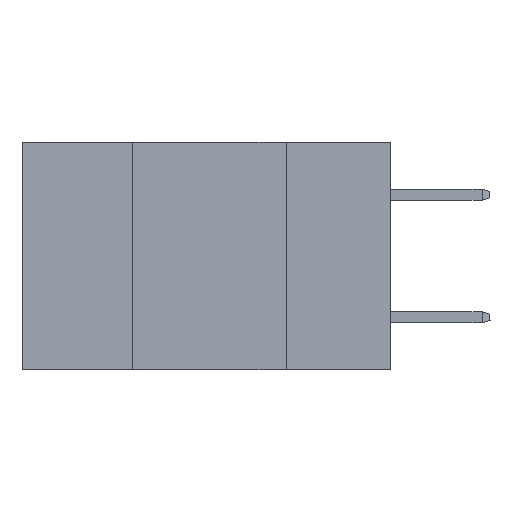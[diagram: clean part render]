
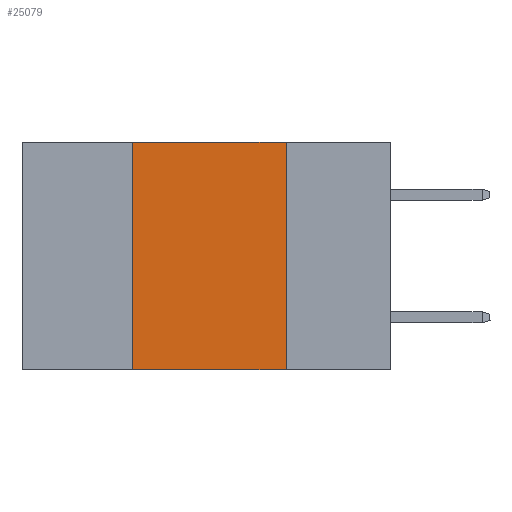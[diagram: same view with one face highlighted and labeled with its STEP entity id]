
A CAD part, left-side view. The second image highlights one B-rep face of the part: STEP entity #25079.
In plain terms, the highlighted planar face has unit normal (-1, 0, 0).
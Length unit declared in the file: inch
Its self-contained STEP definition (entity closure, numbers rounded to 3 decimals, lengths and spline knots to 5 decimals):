
#1351 = ORIENTED_EDGE ( 'NONE', *, *, #25107, .T. ) ;
#2371 = VECTOR ( 'NONE', #12597, 39.37008 ) ;
#2726 = PLANE ( 'NONE',  #24938 ) ;
#3390 = DIRECTION ( 'NONE',  ( 0., 0., -1. ) ) ;
#3942 = ORIENTED_EDGE ( 'NONE', *, *, #21817, .F. ) ;
#7204 = CARTESIAN_POINT ( 'NONE',  ( 0., 0.6, 0. ) ) ;
#9148 = DIRECTION ( 'NONE',  ( 0., -1., 0. ) ) ;
#9294 = LINE ( 'NONE', #16383, #20181 ) ;
#9802 = EDGE_LOOP ( 'NONE', ( #15113, #3942, #19496, #1351 ) ) ;
#12597 = DIRECTION ( 'NONE',  ( 0., 0., 1. ) ) ;
#13269 = CARTESIAN_POINT ( 'NONE',  ( 0., 0.6, 0. ) ) ;
#13575 = LINE ( 'NONE', #17907, #27527 ) ;
#14464 = VERTEX_POINT ( 'NONE', #16578 ) ;
#14488 = EDGE_CURVE ( 'NONE', #17779, #22284, #9294, .T. ) ;
#15113 = ORIENTED_EDGE ( 'NONE', *, *, #14488, .F. ) ;
#15718 = DIRECTION ( 'NONE',  ( 1., 0., 0. ) ) ;
#16383 = CARTESIAN_POINT ( 'NONE',  ( 0., 0.17, 0. ) ) ;
#16578 = CARTESIAN_POINT ( 'NONE',  ( 0., 0.42, 0. ) ) ;
#16654 = EDGE_CURVE ( 'NONE', #21016, #14464, #19695, .T. ) ;
#17779 = VERTEX_POINT ( 'NONE', #22684 ) ;
#17907 = CARTESIAN_POINT ( 'NONE',  ( 0., 0.6, -0.37 ) ) ;
#18154 = DIRECTION ( 'NONE',  ( 0., -1., 0. ) ) ;
#19057 = CARTESIAN_POINT ( 'NONE',  ( 0., 0.42, 0. ) ) ;
#19496 = ORIENTED_EDGE ( 'NONE', *, *, #16654, .F. ) ;
#19695 = LINE ( 'NONE', #19057, #2371 ) ;
#19894 = DIRECTION ( 'NONE',  ( 0., 0., -1. ) ) ;
#20000 = CARTESIAN_POINT ( 'NONE',  ( 0., 0.42, -0.37 ) ) ;
#20181 = VECTOR ( 'NONE', #3390, 39.37008 ) ;
#20927 = VECTOR ( 'NONE', #18154, 39.37008 ) ;
#21016 = VERTEX_POINT ( 'NONE', #20000 ) ;
#21817 = EDGE_CURVE ( 'NONE', #14464, #17779, #22950, .T. ) ;
#22284 = VERTEX_POINT ( 'NONE', #25083 ) ;
#22684 = CARTESIAN_POINT ( 'NONE',  ( 0., 0.17, 0. ) ) ;
#22950 = LINE ( 'NONE', #7204, #20927 ) ;
#24938 = AXIS2_PLACEMENT_3D ( 'NONE', #13269, #15718, #19894 ) ;
#25079 = ADVANCED_FACE ( 'NONE', ( #25799 ), #2726, .F. ) ;
#25083 = CARTESIAN_POINT ( 'NONE',  ( 0., 0.17, -0.37 ) ) ;
#25107 = EDGE_CURVE ( 'NONE', #21016, #22284, #13575, .T. ) ;
#25799 = FACE_OUTER_BOUND ( 'NONE', #9802, .T. ) ;
#27527 = VECTOR ( 'NONE', #9148, 39.37008 ) ;
